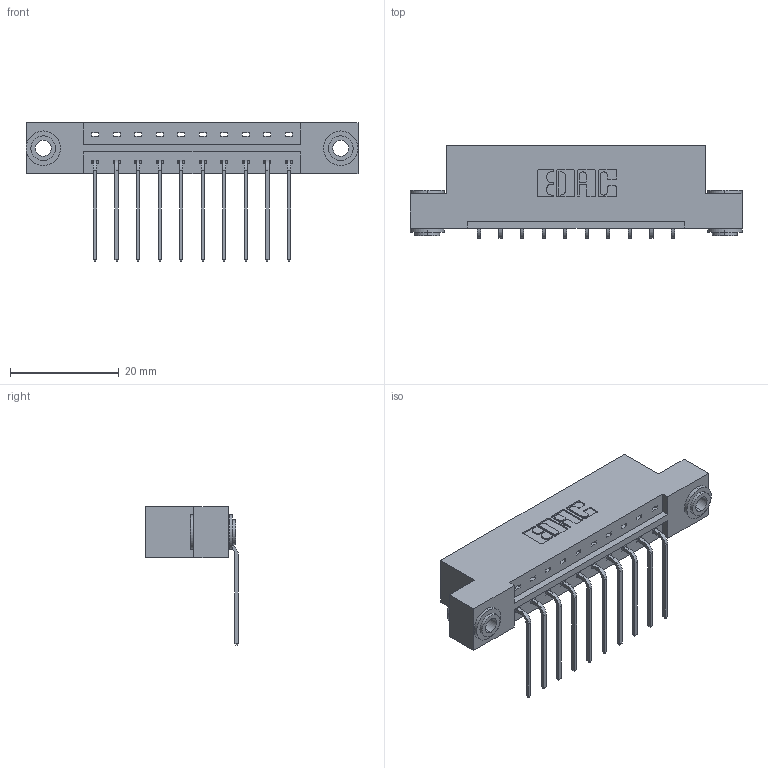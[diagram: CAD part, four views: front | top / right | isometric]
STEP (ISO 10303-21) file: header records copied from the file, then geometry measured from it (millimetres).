
FILE_DESCRIPTION (( 'STEP AP203' ), '1' );
FILE_NAME ('333-010-559-103.STEP', '2018-07-31T23:11:12', ( '' ), ( '' ), 'SwSTEP 2.0', 'SolidWorks 2016', '' );
FILE_SCHEMA (( 'CONFIG_CONTROL_DESIGN' ));
Length unit declared in the file: inch
Products named in the file (4): 333 Part_Flush - .156 Dia - TH; 345-292-001_558 559 Tail - 1; 345-250-002_345-250-002-102; 333-010-559-103
Assembly tree (13 placements, depth 2):
  333-010-559-103
    333 Part_Flush - .156 Dia - TH
    345-292-001_558 559 Tail - 1  x10
    345-250-002_345-250-002-102  x2
Bounding box: 61.16 x 17.09 x 25.53 mm (x, y, z)
Volume: 5932.3 mm3; surface area: 6641 mm2
Topology: 13 solids, 13 shells, 752 faces, 2207 edges, 1454 vertices
Faces by surface type: plane 520, cylinder 224, cone 8
Entity records: 10986 total; most frequent: CARTESIAN_POINT 1879, ORIENTED_EDGE 1818, DIRECTION 1683, EDGE_CURVE 909, VECTOR 757, LINE 757, VERTEX_POINT 602, AXIS2_PLACEMENT_3D 463
